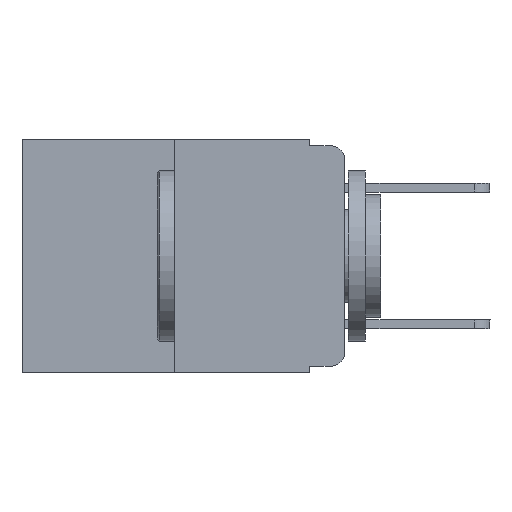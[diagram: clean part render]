
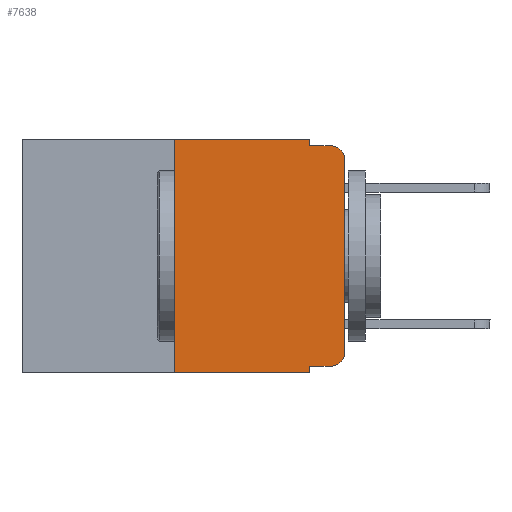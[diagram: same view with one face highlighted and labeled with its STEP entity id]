
A CAD part, left-side view. The second image highlights one B-rep face of the part: STEP entity #7638.
In plain terms, the highlighted planar face has unit normal (-1, 0, 0).
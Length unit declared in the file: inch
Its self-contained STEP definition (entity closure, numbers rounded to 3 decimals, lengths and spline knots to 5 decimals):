
#108 = ORIENTED_EDGE ( 'NONE', *, *, #2213, .F. ) ;
#543 = VECTOR ( 'NONE', #646, 39.37008 ) ;
#646 = DIRECTION ( 'NONE',  ( 0., 0., -1. ) ) ;
#833 = CARTESIAN_POINT ( 'NONE',  ( 0., 0.051, 0. ) ) ;
#943 = DIRECTION ( 'NONE',  ( 0., 0., 1. ) ) ;
#1060 = CARTESIAN_POINT ( 'NONE',  ( 0., 0.02, -0.01 ) ) ;
#1101 = CARTESIAN_POINT ( 'NONE',  ( 0., 0.25, 0. ) ) ;
#1139 = VECTOR ( 'NONE', #943, 39.37008 ) ;
#2093 = CARTESIAN_POINT ( 'NONE',  ( 0., 0., -0.03 ) ) ;
#2213 = EDGE_CURVE ( 'NONE', #12368, #16728, #11103, .T. ) ;
#2423 = CARTESIAN_POINT ( 'NONE',  ( 0., 0.051, 0. ) ) ;
#2667 = DIRECTION ( 'NONE',  ( -1., 0., 0. ) ) ;
#2671 = EDGE_CURVE ( 'NONE', #11207, #16966, #14068, .T. ) ;
#2729 = CARTESIAN_POINT ( 'NONE',  ( 0., 0.02, -0.03 ) ) ;
#2777 = DIRECTION ( 'NONE',  ( 0., -1., 0. ) ) ;
#2857 = CARTESIAN_POINT ( 'NONE',  ( 0., 0.02, -0.333 ) ) ;
#2882 = ORIENTED_EDGE ( 'NONE', *, *, #3469, .F. ) ;
#2953 = CARTESIAN_POINT ( 'NONE',  ( 0., 0.02, -0.313 ) ) ;
#3469 = EDGE_CURVE ( 'NONE', #12165, #9896, #11480, .T. ) ;
#3916 = DIRECTION ( 'NONE',  ( 0., 0., -1. ) ) ;
#4229 = EDGE_CURVE ( 'NONE', #5342, #12165, #12554, .T. ) ;
#4477 = AXIS2_PLACEMENT_3D ( 'NONE', #11365, #11544, #12749 ) ;
#5001 = CARTESIAN_POINT ( 'NONE',  ( 0., 0., 0. ) ) ;
#5079 = EDGE_CURVE ( 'NONE', #12368, #11207, #10802, .T. ) ;
#5302 = EDGE_CURVE ( 'NONE', #6809, #16728, #9751, .T. ) ;
#5342 = VERTEX_POINT ( 'NONE', #2423 ) ;
#5513 = FACE_OUTER_BOUND ( 'NONE', #7700, .T. ) ;
#5582 = EDGE_CURVE ( 'NONE', #12722, #5342, #12505, .T. ) ;
#5647 = CARTESIAN_POINT ( 'NONE',  ( 0., 0.473, 0. ) ) ;
#5836 = DIRECTION ( 'NONE',  ( 0., -1., 0. ) ) ;
#5910 = CARTESIAN_POINT ( 'NONE',  ( 0., 0., -0.313 ) ) ;
#6670 = ORIENTED_EDGE ( 'NONE', *, *, #5302, .T. ) ;
#6803 = ORIENTED_EDGE ( 'NONE', *, *, #5079, .T. ) ;
#6809 = VERTEX_POINT ( 'NONE', #7078 ) ;
#7078 = CARTESIAN_POINT ( 'NONE',  ( 0., 0.25, -0.343 ) ) ;
#7310 = CARTESIAN_POINT ( 'NONE',  ( 0., 0.25, 0. ) ) ;
#7638 = ADVANCED_FACE ( 'NONE', ( #5513 ), #17077, .F. ) ;
#7658 = EDGE_CURVE ( 'NONE', #6809, #12722, #14040, .T. ) ;
#7700 = EDGE_LOOP ( 'NONE', ( #8006, #8282, #2882, #7961, #16323, #8399, #6670, #108, #6803, #14481 ) ) ;
#7830 = CIRCLE ( 'NONE', #15636, 0.02 ) ;
#7961 = ORIENTED_EDGE ( 'NONE', *, *, #4229, .F. ) ;
#8006 = ORIENTED_EDGE ( 'NONE', *, *, #9904, .T. ) ;
#8282 = ORIENTED_EDGE ( 'NONE', *, *, #15494, .T. ) ;
#8399 = ORIENTED_EDGE ( 'NONE', *, *, #7658, .F. ) ;
#9090 = VECTOR ( 'NONE', #2777, 39.37008 ) ;
#9163 = DIRECTION ( 'NONE',  ( 0., -1., 0. ) ) ;
#9751 = LINE ( 'NONE', #15856, #14197 ) ;
#9896 = VERTEX_POINT ( 'NONE', #1060 ) ;
#9904 = EDGE_CURVE ( 'NONE', #16966, #15831, #10755, .T. ) ;
#10755 = LINE ( 'NONE', #5001, #1139 ) ;
#10802 = LINE ( 'NONE', #14017, #11242 ) ;
#11032 = DIRECTION ( 'NONE',  ( 0., 0., -1. ) ) ;
#11103 = LINE ( 'NONE', #14843, #16434 ) ;
#11207 = VERTEX_POINT ( 'NONE', #2857 ) ;
#11242 = VECTOR ( 'NONE', #5836, 39.37008 ) ;
#11365 = CARTESIAN_POINT ( 'NONE',  ( 0., 0.473, 0. ) ) ;
#11480 = LINE ( 'NONE', #16014, #15542 ) ;
#11544 = DIRECTION ( 'NONE',  ( 1., 0., 0. ) ) ;
#11693 = VECTOR ( 'NONE', #16855, 39.37008 ) ;
#12165 = VERTEX_POINT ( 'NONE', #13330 ) ;
#12368 = VERTEX_POINT ( 'NONE', #15393 ) ;
#12502 = CARTESIAN_POINT ( 'NONE',  ( 0., 0.051, -0.343 ) ) ;
#12505 = LINE ( 'NONE', #5647, #9090 ) ;
#12529 = DIRECTION ( 'NONE',  ( -1., 0., 0. ) ) ;
#12554 = LINE ( 'NONE', #833, #543 ) ;
#12722 = VERTEX_POINT ( 'NONE', #1101 ) ;
#12749 = DIRECTION ( 'NONE',  ( 0., 0., -1. ) ) ;
#13330 = CARTESIAN_POINT ( 'NONE',  ( 0., 0.051, -0.01 ) ) ;
#14017 = CARTESIAN_POINT ( 'NONE',  ( 0., 0.051, -0.333 ) ) ;
#14040 = LINE ( 'NONE', #7310, #11693 ) ;
#14068 = CIRCLE ( 'NONE', #16770, 0.02 ) ;
#14197 = VECTOR ( 'NONE', #15917, 39.37008 ) ;
#14481 = ORIENTED_EDGE ( 'NONE', *, *, #2671, .T. ) ;
#14843 = CARTESIAN_POINT ( 'NONE',  ( 0., 0.051, 0. ) ) ;
#15261 = DIRECTION ( 'NONE',  ( 0., 0., -1. ) ) ;
#15393 = CARTESIAN_POINT ( 'NONE',  ( 0., 0.051, -0.333 ) ) ;
#15494 = EDGE_CURVE ( 'NONE', #15831, #9896, #7830, .T. ) ;
#15542 = VECTOR ( 'NONE', #9163, 39.37008 ) ;
#15636 = AXIS2_PLACEMENT_3D ( 'NONE', #2729, #2667, #11032 ) ;
#15831 = VERTEX_POINT ( 'NONE', #2093 ) ;
#15856 = CARTESIAN_POINT ( 'NONE',  ( 0., 0.473, -0.343 ) ) ;
#15917 = DIRECTION ( 'NONE',  ( 0., -1., 0. ) ) ;
#16014 = CARTESIAN_POINT ( 'NONE',  ( 0., 0.051, -0.01 ) ) ;
#16323 = ORIENTED_EDGE ( 'NONE', *, *, #5582, .F. ) ;
#16434 = VECTOR ( 'NONE', #3916, 39.37008 ) ;
#16728 = VERTEX_POINT ( 'NONE', #12502 ) ;
#16770 = AXIS2_PLACEMENT_3D ( 'NONE', #2953, #12529, #15261 ) ;
#16855 = DIRECTION ( 'NONE',  ( 0., 0., 1. ) ) ;
#16966 = VERTEX_POINT ( 'NONE', #5910 ) ;
#17077 = PLANE ( 'NONE',  #4477 ) ;
